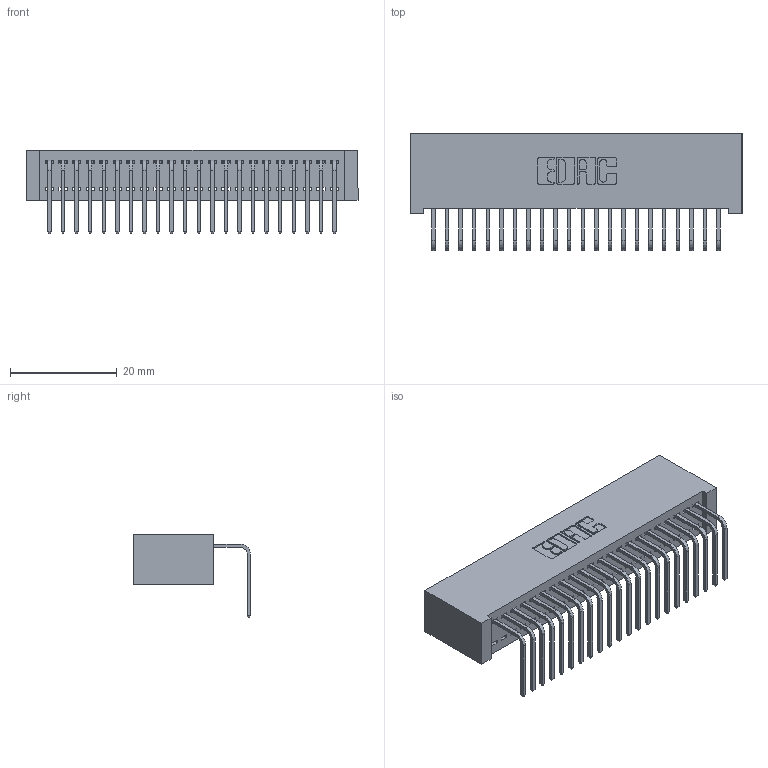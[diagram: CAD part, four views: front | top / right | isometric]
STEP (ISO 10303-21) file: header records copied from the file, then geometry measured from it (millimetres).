
FILE_DESCRIPTION (( 'STEP AP203' ), '1' );
FILE_NAME ('392-022-558-101.STEP', '2018-08-15T13:05:13', ( '' ), ( '' ), 'SwSTEP 2.0', 'SolidWorks 2016', '' );
FILE_SCHEMA (( 'CONFIG_CONTROL_DESIGN' ));
Length unit declared in the file: inch
Products named in the file (3): 342 Part_Lugless; 345-292-001_558 Tail - 2; 392-022-558-101
Assembly tree (23 placements, depth 2):
  392-022-558-101
    342 Part_Lugless
    345-292-001_558 Tail - 2  x22
Bounding box: 62.13 x 21.91 x 15.62 mm (x, y, z)
Volume: 5856 mm3; surface area: 8965.5 mm2
Topology: 23 solids, 23 shells, 1422 faces, 4279 edges, 2822 vertices
Faces by surface type: plane 1030, cylinder 392
Entity records: 15711 total; most frequent: CARTESIAN_POINT 2720, ORIENTED_EDGE 2678, DIRECTION 2327, EDGE_CURVE 1339, LINE 1219, VECTOR 1219, VERTEX_POINT 890, AXIS2_PLACEMENT_3D 554
